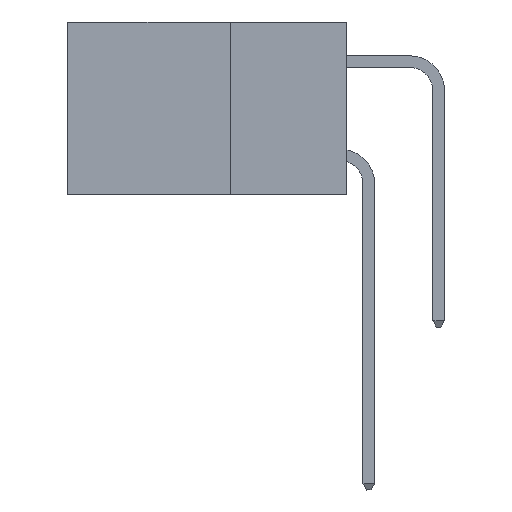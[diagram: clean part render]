
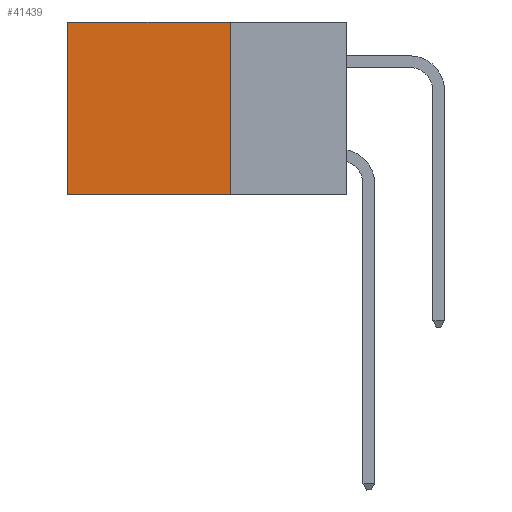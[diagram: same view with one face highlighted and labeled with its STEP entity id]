
A CAD part, left-side view. The second image highlights one B-rep face of the part: STEP entity #41439.
In plain terms, the highlighted planar face has unit normal (-1, 0, 0).
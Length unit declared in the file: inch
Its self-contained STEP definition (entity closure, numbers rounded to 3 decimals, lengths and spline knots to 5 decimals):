
#1429 = FACE_OUTER_BOUND ( 'NONE', #37012, .T. ) ;
#1679 = ORIENTED_EDGE ( 'NONE', *, *, #17324, .T. ) ;
#2009 = VECTOR ( 'NONE', #39549, 39.37008 ) ;
#2411 = DIRECTION ( 'NONE',  ( 0., 1., 0. ) ) ;
#5335 = CARTESIAN_POINT ( 'NONE',  ( 0.2875, 0.25, 0. ) ) ;
#7040 = VECTOR ( 'NONE', #38025, 39.37008 ) ;
#7466 = VERTEX_POINT ( 'NONE', #14458 ) ;
#7554 = VERTEX_POINT ( 'NONE', #32904 ) ;
#9394 = CARTESIAN_POINT ( 'NONE',  ( 0.2875, 0.25, -0.37 ) ) ;
#10092 = AXIS2_PLACEMENT_3D ( 'NONE', #5335, #40126, #15796 ) ;
#10551 = ORIENTED_EDGE ( 'NONE', *, *, #41725, .F. ) ;
#11354 = LINE ( 'NONE', #32586, #2009 ) ;
#14458 = CARTESIAN_POINT ( 'NONE',  ( 0.2875, 0.25, -0.37 ) ) ;
#14971 = ORIENTED_EDGE ( 'NONE', *, *, #17712, .F. ) ;
#15796 = DIRECTION ( 'NONE',  ( 0., 0., -1. ) ) ;
#16240 = VECTOR ( 'NONE', #2411, 39.37008 ) ;
#17324 = EDGE_CURVE ( 'NONE', #19277, #26879, #11354, .T. ) ;
#17712 = EDGE_CURVE ( 'NONE', #7466, #26879, #18475, .T. ) ;
#18324 = EDGE_CURVE ( 'NONE', #7554, #19277, #35463, .T. ) ;
#18475 = LINE ( 'NONE', #9394, #43854 ) ;
#19156 = PLANE ( 'NONE',  #10092 ) ;
#19277 = VERTEX_POINT ( 'NONE', #44852 ) ;
#20421 = DIRECTION ( 'NONE',  ( 0., 1., 0. ) ) ;
#20989 = CARTESIAN_POINT ( 'NONE',  ( 0.2875, 0.25, 0. ) ) ;
#21674 = CARTESIAN_POINT ( 'NONE',  ( 0.2875, 0.6, -0.37 ) ) ;
#21905 = LINE ( 'NONE', #20989, #7040 ) ;
#26879 = VERTEX_POINT ( 'NONE', #21674 ) ;
#27311 = CARTESIAN_POINT ( 'NONE',  ( 0.2875, 0.25, 0. ) ) ;
#32586 = CARTESIAN_POINT ( 'NONE',  ( 0.2875, 0.6, 0. ) ) ;
#32904 = CARTESIAN_POINT ( 'NONE',  ( 0.2875, 0.25, 0. ) ) ;
#35463 = LINE ( 'NONE', #27311, #16240 ) ;
#37012 = EDGE_LOOP ( 'NONE', ( #1679, #14971, #10551, #40347 ) ) ;
#38025 = DIRECTION ( 'NONE',  ( 0., 0., -1. ) ) ;
#39549 = DIRECTION ( 'NONE',  ( 0., 0., -1. ) ) ;
#40126 = DIRECTION ( 'NONE',  ( 1., 0., 0. ) ) ;
#40347 = ORIENTED_EDGE ( 'NONE', *, *, #18324, .T. ) ;
#41439 = ADVANCED_FACE ( 'NONE', ( #1429 ), #19156, .F. ) ;
#41725 = EDGE_CURVE ( 'NONE', #7554, #7466, #21905, .T. ) ;
#43854 = VECTOR ( 'NONE', #20421, 39.37008 ) ;
#44852 = CARTESIAN_POINT ( 'NONE',  ( 0.2875, 0.6, 0. ) ) ;
